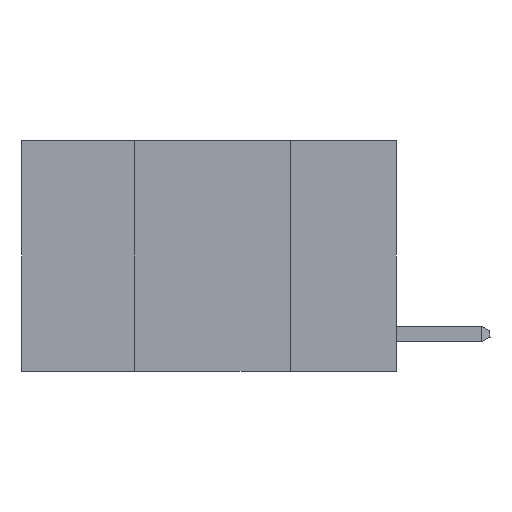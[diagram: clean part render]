
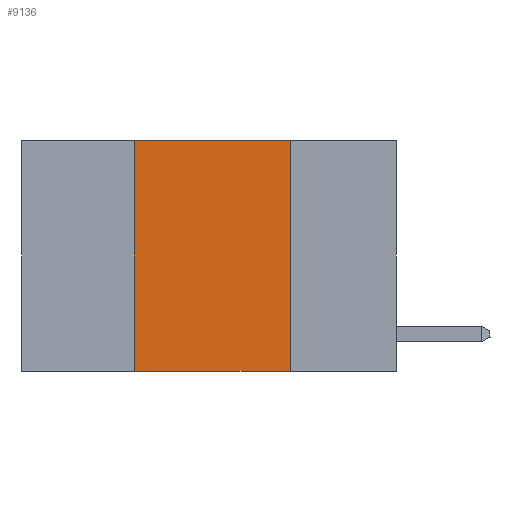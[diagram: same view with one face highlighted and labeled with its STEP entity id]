
A CAD part, left-side view. The second image highlights one B-rep face of the part: STEP entity #9136.
In plain terms, the highlighted planar face has unit normal (-1, 0, 0).
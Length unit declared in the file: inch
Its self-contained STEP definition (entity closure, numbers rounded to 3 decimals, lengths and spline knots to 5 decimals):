
#232 = CARTESIAN_POINT ( 'NONE',  ( 0., 0.6, 0. ) ) ;
#448 = EDGE_LOOP ( 'NONE', ( #9351, #768, #11655, #11583 ) ) ;
#750 = DIRECTION ( 'NONE',  ( 0., -1., 0. ) ) ;
#768 = ORIENTED_EDGE ( 'NONE', *, *, #5642, .F. ) ;
#1013 = CARTESIAN_POINT ( 'NONE',  ( 0., 0.42, 0. ) ) ;
#1222 = PLANE ( 'NONE',  #10260 ) ;
#2085 = LINE ( 'NONE', #4238, #4069 ) ;
#2086 = DIRECTION ( 'NONE',  ( 1., 0., 0. ) ) ;
#2244 = LINE ( 'NONE', #232, #4795 ) ;
#2597 = DIRECTION ( 'NONE',  ( 0., 0., 1. ) ) ;
#3093 = VECTOR ( 'NONE', #10518, 39.37008 ) ;
#3383 = DIRECTION ( 'NONE',  ( 0., -1., 0. ) ) ;
#3714 = CARTESIAN_POINT ( 'NONE',  ( 0., 0.6, 0. ) ) ;
#4069 = VECTOR ( 'NONE', #3383, 39.37008 ) ;
#4105 = CARTESIAN_POINT ( 'NONE',  ( 0., 0.42, -0.37 ) ) ;
#4238 = CARTESIAN_POINT ( 'NONE',  ( 0., 0.6, -0.37 ) ) ;
#4308 = CARTESIAN_POINT ( 'NONE',  ( 0., 0.17, -0.37 ) ) ;
#4795 = VECTOR ( 'NONE', #750, 39.37008 ) ;
#4855 = CARTESIAN_POINT ( 'NONE',  ( 0., 0.17, 0. ) ) ;
#5247 = VERTEX_POINT ( 'NONE', #4105 ) ;
#5642 = EDGE_CURVE ( 'NONE', #7463, #7974, #2244, .T. ) ;
#6478 = EDGE_CURVE ( 'NONE', #5247, #7033, #2085, .T. ) ;
#6496 = EDGE_CURVE ( 'NONE', #5247, #7463, #11182, .T. ) ;
#7033 = VERTEX_POINT ( 'NONE', #4308 ) ;
#7354 = EDGE_CURVE ( 'NONE', #7974, #7033, #10756, .T. ) ;
#7463 = VERTEX_POINT ( 'NONE', #1013 ) ;
#7974 = VERTEX_POINT ( 'NONE', #4855 ) ;
#8454 = DIRECTION ( 'NONE',  ( 0., 0., -1. ) ) ;
#8500 = VECTOR ( 'NONE', #2597, 39.37008 ) ;
#9136 = ADVANCED_FACE ( 'NONE', ( #11464 ), #1222, .F. ) ;
#9351 = ORIENTED_EDGE ( 'NONE', *, *, #7354, .F. ) ;
#10007 = CARTESIAN_POINT ( 'NONE',  ( 0., 0.42, 0. ) ) ;
#10260 = AXIS2_PLACEMENT_3D ( 'NONE', #3714, #2086, #8454 ) ;
#10518 = DIRECTION ( 'NONE',  ( 0., 0., -1. ) ) ;
#10558 = CARTESIAN_POINT ( 'NONE',  ( 0., 0.17, 0. ) ) ;
#10756 = LINE ( 'NONE', #10558, #3093 ) ;
#11182 = LINE ( 'NONE', #10007, #8500 ) ;
#11464 = FACE_OUTER_BOUND ( 'NONE', #448, .T. ) ;
#11583 = ORIENTED_EDGE ( 'NONE', *, *, #6478, .T. ) ;
#11655 = ORIENTED_EDGE ( 'NONE', *, *, #6496, .F. ) ;
